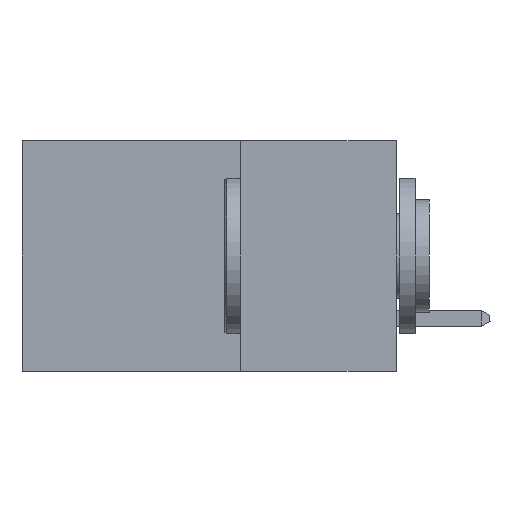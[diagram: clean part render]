
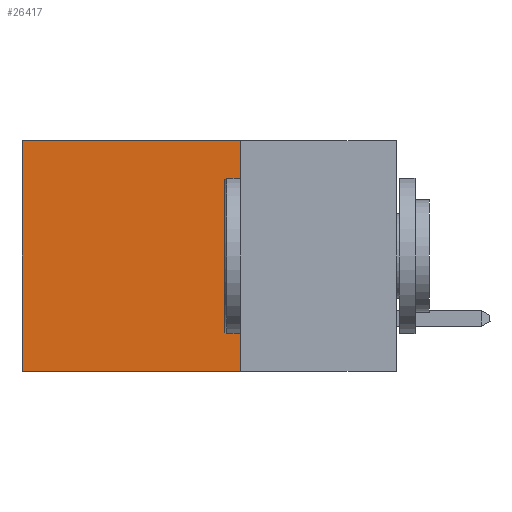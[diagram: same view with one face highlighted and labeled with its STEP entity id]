
A CAD part, left-side view. The second image highlights one B-rep face of the part: STEP entity #26417.
In plain terms, the highlighted planar face has unit normal (-1, 0, 0).
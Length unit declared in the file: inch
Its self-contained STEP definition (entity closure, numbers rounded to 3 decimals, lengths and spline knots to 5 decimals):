
#893 = CARTESIAN_POINT ( 'NONE',  ( 0.298, 0.25, 0. ) ) ;
#2393 = CARTESIAN_POINT ( 'NONE',  ( 0.298, 0.25, 0. ) ) ;
#3620 = CARTESIAN_POINT ( 'NONE',  ( 0.298, 0.6, 0. ) ) ;
#3740 = EDGE_CURVE ( 'NONE', #16493, #10159, #5247, .T. ) ;
#3865 = DIRECTION ( 'NONE',  ( 0., 1., 0. ) ) ;
#4461 = LINE ( 'NONE', #3620, #18358 ) ;
#4838 = CARTESIAN_POINT ( 'NONE',  ( 0.298, 0.6, -0.37 ) ) ;
#5247 = LINE ( 'NONE', #13712, #14907 ) ;
#6719 = VECTOR ( 'NONE', #17929, 39.37008 ) ;
#7783 = CARTESIAN_POINT ( 'NONE',  ( 0.298, 0.25, 0. ) ) ;
#9350 = ORIENTED_EDGE ( 'NONE', *, *, #16912, .F. ) ;
#9638 = VERTEX_POINT ( 'NONE', #2393 ) ;
#10159 = VERTEX_POINT ( 'NONE', #4838 ) ;
#11330 = CARTESIAN_POINT ( 'NONE',  ( 0.298, 0.25, -0.37 ) ) ;
#12511 = LINE ( 'NONE', #16866, #6719 ) ;
#13712 = CARTESIAN_POINT ( 'NONE',  ( 0.298, 0.25, -0.37 ) ) ;
#14907 = VECTOR ( 'NONE', #3865, 39.37008 ) ;
#15371 = ORIENTED_EDGE ( 'NONE', *, *, #16257, .T. ) ;
#16257 = EDGE_CURVE ( 'NONE', #29398, #10159, #4461, .T. ) ;
#16493 = VERTEX_POINT ( 'NONE', #11330 ) ;
#16866 = CARTESIAN_POINT ( 'NONE',  ( 0.298, 0.25, 0. ) ) ;
#16912 = EDGE_CURVE ( 'NONE', #9638, #16493, #12511, .T. ) ;
#17670 = CARTESIAN_POINT ( 'NONE',  ( 0.298, 0.6, 0. ) ) ;
#17710 = DIRECTION ( 'NONE',  ( 0., 1., 0. ) ) ;
#17929 = DIRECTION ( 'NONE',  ( 0., 0., -1. ) ) ;
#18358 = VECTOR ( 'NONE', #30888, 39.37008 ) ;
#22212 = ORIENTED_EDGE ( 'NONE', *, *, #24607, .T. ) ;
#22887 = PLANE ( 'NONE',  #31556 ) ;
#24562 = ORIENTED_EDGE ( 'NONE', *, *, #3740, .F. ) ;
#24607 = EDGE_CURVE ( 'NONE', #9638, #29398, #27466, .T. ) ;
#24730 = FACE_OUTER_BOUND ( 'NONE', #26377, .T. ) ;
#25360 = DIRECTION ( 'NONE',  ( 0., 0., -1. ) ) ;
#25674 = DIRECTION ( 'NONE',  ( 1., 0., 0. ) ) ;
#26377 = EDGE_LOOP ( 'NONE', ( #15371, #24562, #9350, #22212 ) ) ;
#26417 = ADVANCED_FACE ( 'NONE', ( #24730 ), #22887, .F. ) ;
#27093 = VECTOR ( 'NONE', #17710, 39.37008 ) ;
#27466 = LINE ( 'NONE', #7783, #27093 ) ;
#29398 = VERTEX_POINT ( 'NONE', #17670 ) ;
#30888 = DIRECTION ( 'NONE',  ( 0., 0., -1. ) ) ;
#31556 = AXIS2_PLACEMENT_3D ( 'NONE', #893, #25674, #25360 ) ;
